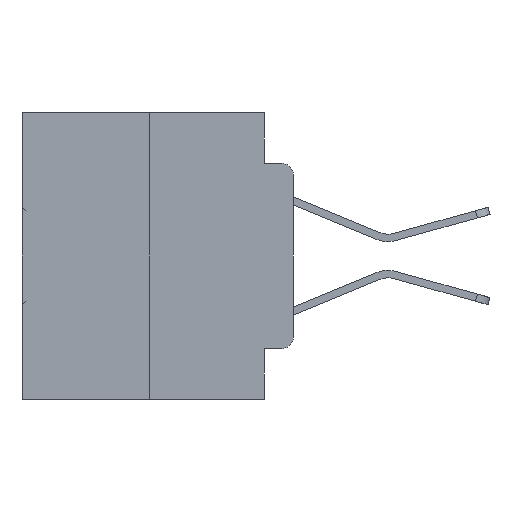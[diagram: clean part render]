
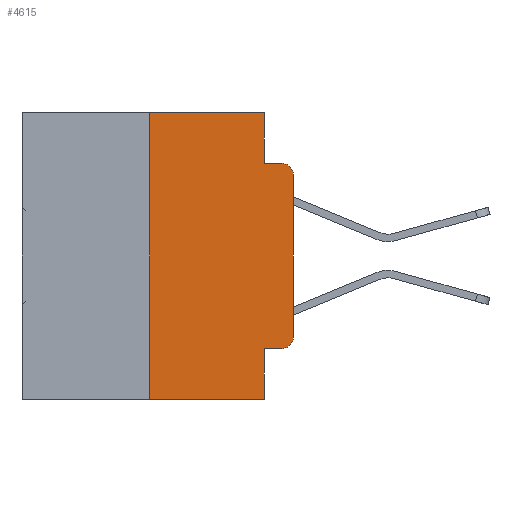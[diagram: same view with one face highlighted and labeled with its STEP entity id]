
A CAD part, left-side view. The second image highlights one B-rep face of the part: STEP entity #4615.
In plain terms, the highlighted planar face has unit normal (-1, 0, 0).
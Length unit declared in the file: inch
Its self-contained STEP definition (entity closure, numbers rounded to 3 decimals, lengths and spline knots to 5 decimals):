
#101 = ORIENTED_EDGE ( 'NONE', *, *, #11294, .F. ) ;
#113 = CARTESIAN_POINT ( 'NONE',  ( 0., 0.051, 0. ) ) ;
#629 = CARTESIAN_POINT ( 'NONE',  ( 0., 0., -0.3915 ) ) ;
#951 = CARTESIAN_POINT ( 'NONE',  ( 0., 0.051, -0.4115 ) ) ;
#1680 = VERTEX_POINT ( 'NONE', #10447 ) ;
#1723 = VECTOR ( 'NONE', #21523, 39.37008 ) ;
#1745 = ORIENTED_EDGE ( 'NONE', *, *, #29046, .F. ) ;
#1820 = CARTESIAN_POINT ( 'NONE',  ( 0., 0.051, -0.4115 ) ) ;
#2002 = DIRECTION ( 'NONE',  ( 1., 0., 0. ) ) ;
#2133 = ORIENTED_EDGE ( 'NONE', *, *, #7951, .T. ) ;
#2190 = PLANE ( 'NONE',  #28768 ) ;
#2473 = CIRCLE ( 'NONE', #23849, 0.02 ) ;
#2528 = CARTESIAN_POINT ( 'NONE',  ( 0., 0.25, -0.5 ) ) ;
#3445 = VECTOR ( 'NONE', #16846, 39.37008 ) ;
#3689 = DIRECTION ( 'NONE',  ( 0., 0., -1. ) ) ;
#4230 = CARTESIAN_POINT ( 'NONE',  ( 0., 0.473, -0.5 ) ) ;
#4429 = DIRECTION ( 'NONE',  ( 0., 0., -1. ) ) ;
#4588 = CARTESIAN_POINT ( 'NONE',  ( 0., 0.473, 0. ) ) ;
#4615 = ADVANCED_FACE ( 'NONE', ( #19996 ), #2190, .F. ) ;
#4660 = VERTEX_POINT ( 'NONE', #2528 ) ;
#5104 = VECTOR ( 'NONE', #31527, 39.37008 ) ;
#5246 = VERTEX_POINT ( 'NONE', #11181 ) ;
#6419 = CARTESIAN_POINT ( 'NONE',  ( 0., 0.051, -0.0885 ) ) ;
#7951 = EDGE_CURVE ( 'NONE', #8599, #20991, #2473, .T. ) ;
#7992 = ORIENTED_EDGE ( 'NONE', *, *, #24717, .T. ) ;
#8599 = VERTEX_POINT ( 'NONE', #23481 ) ;
#8987 = EDGE_CURVE ( 'NONE', #16114, #1680, #25435, .T. ) ;
#10335 = ORIENTED_EDGE ( 'NONE', *, *, #27189, .F. ) ;
#10447 = CARTESIAN_POINT ( 'NONE',  ( 0., 0.051, -0.0885 ) ) ;
#10909 = LINE ( 'NONE', #28674, #30140 ) ;
#11181 = CARTESIAN_POINT ( 'NONE',  ( 0., 0.25, 0. ) ) ;
#11264 = CARTESIAN_POINT ( 'NONE',  ( 0., 0.473, 0. ) ) ;
#11294 = EDGE_CURVE ( 'NONE', #4660, #5246, #25353, .T. ) ;
#11398 = CARTESIAN_POINT ( 'NONE',  ( 0., 0.02, -0.4115 ) ) ;
#11403 = CARTESIAN_POINT ( 'NONE',  ( 0., 0.02, -0.1085 ) ) ;
#11519 = DIRECTION ( 'NONE',  ( 0., -1., 0. ) ) ;
#12144 = VERTEX_POINT ( 'NONE', #23087 ) ;
#12628 = ORIENTED_EDGE ( 'NONE', *, *, #20239, .F. ) ;
#12980 = LINE ( 'NONE', #6419, #31433 ) ;
#13574 = CARTESIAN_POINT ( 'NONE',  ( 0., 0.02, -0.3915 ) ) ;
#13813 = DIRECTION ( 'NONE',  ( 0., 0., -1. ) ) ;
#14119 = DIRECTION ( 'NONE',  ( 0., 0., 1. ) ) ;
#15030 = DIRECTION ( 'NONE',  ( 0., 0., -1. ) ) ;
#16040 = DIRECTION ( 'NONE',  ( 0., 0., -1. ) ) ;
#16114 = VERTEX_POINT ( 'NONE', #21455 ) ;
#16267 = CIRCLE ( 'NONE', #19430, 0.02 ) ;
#16846 = DIRECTION ( 'NONE',  ( 0., -1., 0. ) ) ;
#19430 = AXIS2_PLACEMENT_3D ( 'NONE', #13574, #30408, #16040 ) ;
#19996 = FACE_OUTER_BOUND ( 'NONE', #20758, .T. ) ;
#20239 = EDGE_CURVE ( 'NONE', #5246, #16114, #28606, .T. ) ;
#20356 = LINE ( 'NONE', #30939, #26015 ) ;
#20652 = ORIENTED_EDGE ( 'NONE', *, *, #25468, .T. ) ;
#20758 = EDGE_LOOP ( 'NONE', ( #7992, #2133, #10335, #31069, #12628, #101, #20652, #1745, #21849, #29681 ) ) ;
#20991 = VERTEX_POINT ( 'NONE', #27038 ) ;
#21379 = LINE ( 'NONE', #1820, #1723 ) ;
#21455 = CARTESIAN_POINT ( 'NONE',  ( 0., 0.051, 0. ) ) ;
#21523 = DIRECTION ( 'NONE',  ( 0., -1., 0. ) ) ;
#21849 = ORIENTED_EDGE ( 'NONE', *, *, #22047, .T. ) ;
#22047 = EDGE_CURVE ( 'NONE', #23228, #24628, #21379, .T. ) ;
#23087 = CARTESIAN_POINT ( 'NONE',  ( 0., 0.051, -0.5 ) ) ;
#23228 = VERTEX_POINT ( 'NONE', #951 ) ;
#23274 = EDGE_CURVE ( 'NONE', #24628, #28711, #16267, .T. ) ;
#23481 = CARTESIAN_POINT ( 'NONE',  ( 0., 0., -0.1085 ) ) ;
#23814 = DIRECTION ( 'NONE',  ( 0., -1., 0. ) ) ;
#23849 = AXIS2_PLACEMENT_3D ( 'NONE', #11403, #28275, #13813 ) ;
#24380 = CARTESIAN_POINT ( 'NONE',  ( 0., 0.25, 0. ) ) ;
#24628 = VERTEX_POINT ( 'NONE', #11398 ) ;
#24717 = EDGE_CURVE ( 'NONE', #28711, #8599, #20356, .T. ) ;
#25353 = LINE ( 'NONE', #24380, #5104 ) ;
#25435 = LINE ( 'NONE', #113, #30960 ) ;
#25468 = EDGE_CURVE ( 'NONE', #4660, #12144, #30376, .T. ) ;
#26015 = VECTOR ( 'NONE', #14119, 39.37008 ) ;
#27038 = CARTESIAN_POINT ( 'NONE',  ( 0., 0.02, -0.0885 ) ) ;
#27189 = EDGE_CURVE ( 'NONE', #1680, #20991, #12980, .T. ) ;
#28275 = DIRECTION ( 'NONE',  ( -1., 0., 0. ) ) ;
#28606 = LINE ( 'NONE', #4588, #3445 ) ;
#28674 = CARTESIAN_POINT ( 'NONE',  ( 0., 0.051, 0. ) ) ;
#28711 = VERTEX_POINT ( 'NONE', #629 ) ;
#28768 = AXIS2_PLACEMENT_3D ( 'NONE', #11264, #2002, #3689 ) ;
#29046 = EDGE_CURVE ( 'NONE', #23228, #12144, #10909, .T. ) ;
#29640 = VECTOR ( 'NONE', #23814, 39.37008 ) ;
#29681 = ORIENTED_EDGE ( 'NONE', *, *, #23274, .T. ) ;
#30140 = VECTOR ( 'NONE', #4429, 39.37008 ) ;
#30376 = LINE ( 'NONE', #4230, #29640 ) ;
#30408 = DIRECTION ( 'NONE',  ( -1., 0., 0. ) ) ;
#30939 = CARTESIAN_POINT ( 'NONE',  ( 0., 0., 0. ) ) ;
#30960 = VECTOR ( 'NONE', #15030, 39.37008 ) ;
#31069 = ORIENTED_EDGE ( 'NONE', *, *, #8987, .F. ) ;
#31433 = VECTOR ( 'NONE', #11519, 39.37008 ) ;
#31527 = DIRECTION ( 'NONE',  ( 0., 0., 1. ) ) ;
